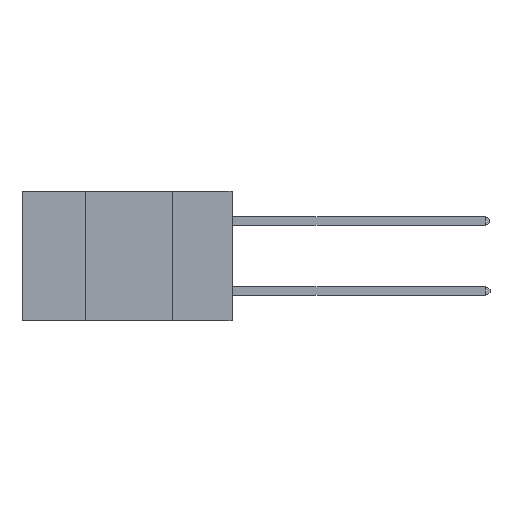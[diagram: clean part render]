
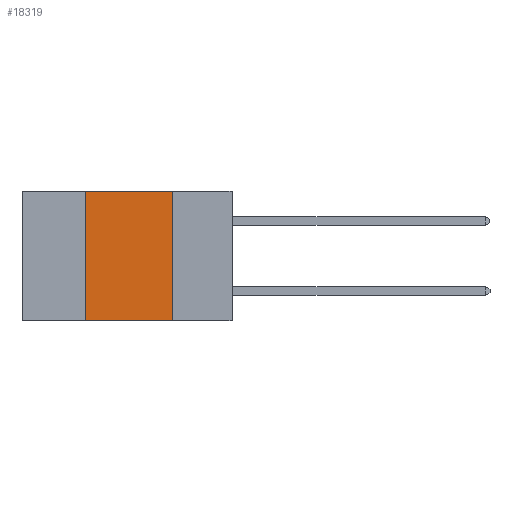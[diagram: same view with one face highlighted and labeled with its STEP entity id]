
A CAD part, left-side view. The second image highlights one B-rep face of the part: STEP entity #18319.
In plain terms, the highlighted planar face has unit normal (-1, 0, 0).
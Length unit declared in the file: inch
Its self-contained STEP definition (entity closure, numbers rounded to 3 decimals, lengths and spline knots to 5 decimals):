
#421 = VERTEX_POINT ( 'NONE', #6140 ) ;
#1062 = VECTOR ( 'NONE', #12644, 39.37008 ) ;
#1786 = EDGE_CURVE ( 'NONE', #12845, #421, #17526, .T. ) ;
#2166 = DIRECTION ( 'NONE',  ( 0., 0., 1. ) ) ;
#2559 = CARTESIAN_POINT ( 'NONE',  ( 0., 0.42, 0. ) ) ;
#2682 = AXIS2_PLACEMENT_3D ( 'NONE', #4589, #14920, #6090 ) ;
#2881 = EDGE_CURVE ( 'NONE', #17574, #12845, #8625, .T. ) ;
#2957 = ORIENTED_EDGE ( 'NONE', *, *, #2881, .F. ) ;
#3442 = ORIENTED_EDGE ( 'NONE', *, *, #14294, .T. ) ;
#4589 = CARTESIAN_POINT ( 'NONE',  ( 0., 0.6, 0. ) ) ;
#5045 = VECTOR ( 'NONE', #18264, 39.37008 ) ;
#6090 = DIRECTION ( 'NONE',  ( 0., 0., -1. ) ) ;
#6140 = CARTESIAN_POINT ( 'NONE',  ( 0., 0.17, -0.37 ) ) ;
#6421 = LINE ( 'NONE', #11209, #14263 ) ;
#6533 = EDGE_CURVE ( 'NONE', #15939, #17574, #6421, .T. ) ;
#6955 = ORIENTED_EDGE ( 'NONE', *, *, #6533, .F. ) ;
#7537 = DIRECTION ( 'NONE',  ( 0., 0., -1. ) ) ;
#7800 = CARTESIAN_POINT ( 'NONE',  ( 0., 0.17, 0. ) ) ;
#8625 = LINE ( 'NONE', #12436, #5045 ) ;
#11209 = CARTESIAN_POINT ( 'NONE',  ( 0., 0.42, 0. ) ) ;
#11949 = CARTESIAN_POINT ( 'NONE',  ( 0., 0.42, -0.37 ) ) ;
#12436 = CARTESIAN_POINT ( 'NONE',  ( 0., 0.6, 0. ) ) ;
#12644 = DIRECTION ( 'NONE',  ( 0., -1., 0. ) ) ;
#12845 = VERTEX_POINT ( 'NONE', #14534 ) ;
#13458 = PLANE ( 'NONE',  #2682 ) ;
#13602 = VECTOR ( 'NONE', #7537, 39.37008 ) ;
#14075 = CARTESIAN_POINT ( 'NONE',  ( 0., 0.6, -0.37 ) ) ;
#14263 = VECTOR ( 'NONE', #2166, 39.37008 ) ;
#14277 = FACE_OUTER_BOUND ( 'NONE', #18986, .T. ) ;
#14294 = EDGE_CURVE ( 'NONE', #15939, #421, #16938, .T. ) ;
#14534 = CARTESIAN_POINT ( 'NONE',  ( 0., 0.17, 0. ) ) ;
#14920 = DIRECTION ( 'NONE',  ( 1., 0., 0. ) ) ;
#15939 = VERTEX_POINT ( 'NONE', #11949 ) ;
#16938 = LINE ( 'NONE', #14075, #1062 ) ;
#17526 = LINE ( 'NONE', #7800, #13602 ) ;
#17574 = VERTEX_POINT ( 'NONE', #2559 ) ;
#17774 = ORIENTED_EDGE ( 'NONE', *, *, #1786, .F. ) ;
#18264 = DIRECTION ( 'NONE',  ( 0., -1., 0. ) ) ;
#18319 = ADVANCED_FACE ( 'NONE', ( #14277 ), #13458, .F. ) ;
#18986 = EDGE_LOOP ( 'NONE', ( #17774, #2957, #6955, #3442 ) ) ;
